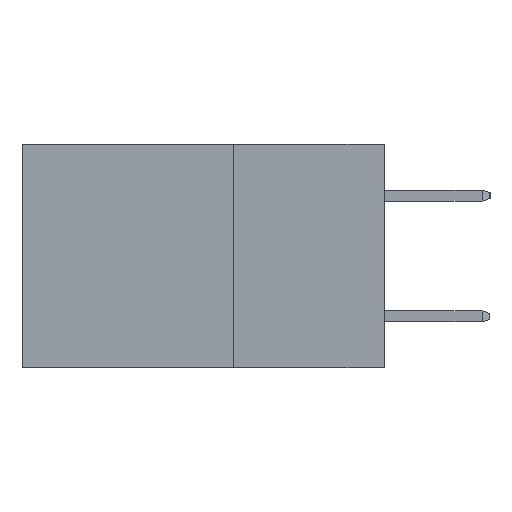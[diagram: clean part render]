
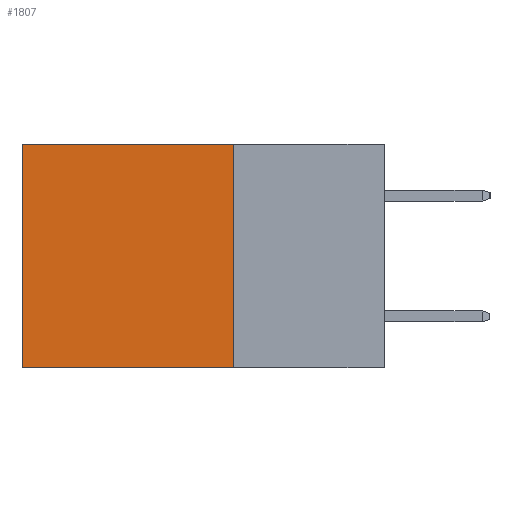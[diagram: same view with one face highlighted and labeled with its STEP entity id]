
A CAD part, left-side view. The second image highlights one B-rep face of the part: STEP entity #1807.
In plain terms, the highlighted planar face has unit normal (-1, 0, 0).
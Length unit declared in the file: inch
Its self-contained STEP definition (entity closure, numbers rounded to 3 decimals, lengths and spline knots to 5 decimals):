
#648 = EDGE_CURVE ( 'NONE', #6016, #2642, #5067, .T. ) ;
#826 = CARTESIAN_POINT ( 'NONE',  ( 0.298, 0.25, 0. ) ) ;
#944 = VERTEX_POINT ( 'NONE', #3735 ) ;
#1597 = EDGE_CURVE ( 'NONE', #2642, #944, #5032, .T. ) ;
#1659 = LINE ( 'NONE', #8716, #4564 ) ;
#1796 = EDGE_LOOP ( 'NONE', ( #8926, #9900, #10144, #7306 ) ) ;
#1807 = ADVANCED_FACE ( 'NONE', ( #10627 ), #3785, .F. ) ;
#2642 = VERTEX_POINT ( 'NONE', #8512 ) ;
#3735 = CARTESIAN_POINT ( 'NONE',  ( 0.298, 0.6, -0.37 ) ) ;
#3785 = PLANE ( 'NONE',  #10254 ) ;
#4060 = VERTEX_POINT ( 'NONE', #6047 ) ;
#4391 = VECTOR ( 'NONE', #10040, 39.37008 ) ;
#4564 = VECTOR ( 'NONE', #6646, 39.37008 ) ;
#4739 = VECTOR ( 'NONE', #5989, 39.37008 ) ;
#4828 = EDGE_CURVE ( 'NONE', #4060, #944, #1659, .T. ) ;
#5032 = LINE ( 'NONE', #5884, #4739 ) ;
#5067 = LINE ( 'NONE', #6388, #9224 ) ;
#5215 = CARTESIAN_POINT ( 'NONE',  ( 0.298, 0.25, 0. ) ) ;
#5884 = CARTESIAN_POINT ( 'NONE',  ( 0.298, 0.6, 0. ) ) ;
#5989 = DIRECTION ( 'NONE',  ( 0., 0., -1. ) ) ;
#6016 = VERTEX_POINT ( 'NONE', #7212 ) ;
#6047 = CARTESIAN_POINT ( 'NONE',  ( 0.298, 0.25, -0.37 ) ) ;
#6388 = CARTESIAN_POINT ( 'NONE',  ( 0.298, 0.25, 0. ) ) ;
#6646 = DIRECTION ( 'NONE',  ( 0., 1., 0. ) ) ;
#6673 = EDGE_CURVE ( 'NONE', #6016, #4060, #6750, .T. ) ;
#6750 = LINE ( 'NONE', #5215, #4391 ) ;
#7212 = CARTESIAN_POINT ( 'NONE',  ( 0.298, 0.25, 0. ) ) ;
#7306 = ORIENTED_EDGE ( 'NONE', *, *, #648, .T. ) ;
#7942 = DIRECTION ( 'NONE',  ( 0., 1., 0. ) ) ;
#8506 = DIRECTION ( 'NONE',  ( 1., 0., 0. ) ) ;
#8512 = CARTESIAN_POINT ( 'NONE',  ( 0.298, 0.6, 0. ) ) ;
#8527 = DIRECTION ( 'NONE',  ( 0., 0., -1. ) ) ;
#8716 = CARTESIAN_POINT ( 'NONE',  ( 0.298, 0.25, -0.37 ) ) ;
#8926 = ORIENTED_EDGE ( 'NONE', *, *, #1597, .T. ) ;
#9224 = VECTOR ( 'NONE', #7942, 39.37008 ) ;
#9900 = ORIENTED_EDGE ( 'NONE', *, *, #4828, .F. ) ;
#10040 = DIRECTION ( 'NONE',  ( 0., 0., -1. ) ) ;
#10144 = ORIENTED_EDGE ( 'NONE', *, *, #6673, .F. ) ;
#10254 = AXIS2_PLACEMENT_3D ( 'NONE', #826, #8506, #8527 ) ;
#10627 = FACE_OUTER_BOUND ( 'NONE', #1796, .T. ) ;
